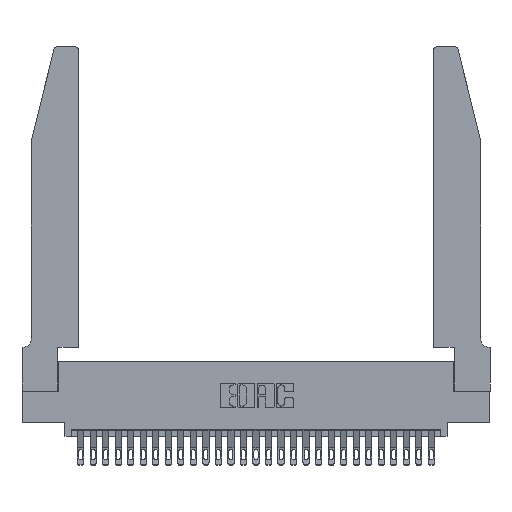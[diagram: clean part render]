
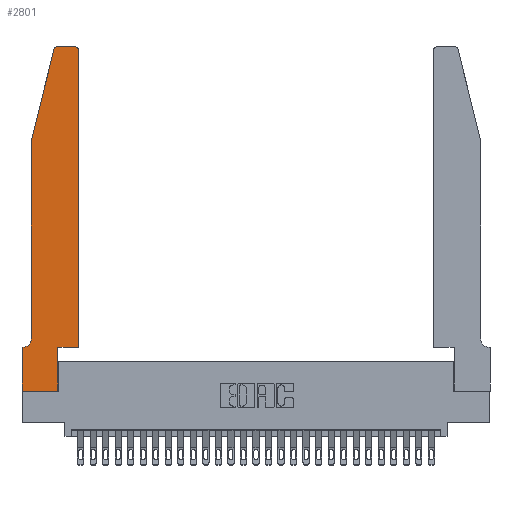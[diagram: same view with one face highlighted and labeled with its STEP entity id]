
A CAD part, top view. The second image highlights one B-rep face of the part: STEP entity #2801.
In plain terms, the highlighted planar face has unit normal (0, 0, 1).
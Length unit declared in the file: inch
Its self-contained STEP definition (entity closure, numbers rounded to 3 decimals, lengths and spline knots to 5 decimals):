
#7 = ORIENTED_EDGE ( 'NONE', *, *, #25601, .T. ) ;
#226 = LINE ( 'NONE', #25525, #24076 ) ;
#768 = ORIENTED_EDGE ( 'NONE', *, *, #28300, .T. ) ;
#838 = LINE ( 'NONE', #29367, #18623 ) ;
#1245 = VERTEX_POINT ( 'NONE', #4473 ) ;
#1294 = CARTESIAN_POINT ( 'NONE',  ( 0., 0.35, 0.37 ) ) ;
#1443 = ORIENTED_EDGE ( 'NONE', *, *, #9442, .T. ) ;
#1467 = CIRCLE ( 'NONE', #15976, 0.03 ) ;
#1729 = LINE ( 'NONE', #11556, #25465 ) ;
#2020 = VERTEX_POINT ( 'NONE', #29300 ) ;
#2185 = EDGE_CURVE ( 'NONE', #14239, #5493, #1467, .T. ) ;
#2212 = DIRECTION ( 'NONE',  ( 1., 0., 0. ) ) ;
#2456 = LINE ( 'NONE', #15847, #26189 ) ;
#2593 = CARTESIAN_POINT ( 'NONE',  ( 0.0055, 0.35, 0.37 ) ) ;
#2801 = ADVANCED_FACE ( 'NONE', ( #16003 ), #4503, .T. ) ;
#2976 = DIRECTION ( 'NONE',  ( -1., 0., 0. ) ) ;
#2997 = CIRCLE ( 'NONE', #26311, 0.07 ) ;
#3949 = DIRECTION ( 'NONE',  ( 0., 1., 0. ) ) ;
#4019 = VERTEX_POINT ( 'NONE', #22606 ) ;
#4306 = ORIENTED_EDGE ( 'NONE', *, *, #5195, .T. ) ;
#4473 = CARTESIAN_POINT ( 'NONE',  ( 0.25487, 2.72718, 0.37 ) ) ;
#4503 = PLANE ( 'NONE',  #16356 ) ;
#4571 = DIRECTION ( 'NONE',  ( 0., 0., -1. ) ) ;
#4838 = DIRECTION ( 'NONE',  ( 0., 0., 1. ) ) ;
#4983 = VECTOR ( 'NONE', #3949, 39.37008 ) ;
#5195 = EDGE_CURVE ( 'NONE', #20004, #14239, #17263, .T. ) ;
#5493 = VERTEX_POINT ( 'NONE', #7193 ) ;
#5931 = CARTESIAN_POINT ( 'NONE',  ( 0.2865, 0., 0.37 ) ) ;
#6699 = DIRECTION ( 'NONE',  ( -1., 0., 0. ) ) ;
#6906 = VERTEX_POINT ( 'NONE', #2593 ) ;
#7050 = DIRECTION ( 'NONE',  ( 1., 0., 0. ) ) ;
#7193 = CARTESIAN_POINT ( 'NONE',  ( 0.4205, 2.75, 0.37 ) ) ;
#7269 = EDGE_CURVE ( 'NONE', #10638, #6906, #2997, .T. ) ;
#8302 = ORIENTED_EDGE ( 'NONE', *, *, #29014, .T. ) ;
#8528 = ORIENTED_EDGE ( 'NONE', *, *, #25649, .T. ) ;
#8791 = DIRECTION ( 'NONE',  ( 0., 0., 1. ) ) ;
#9200 = VERTEX_POINT ( 'NONE', #1294 ) ;
#9442 = EDGE_CURVE ( 'NONE', #28990, #10638, #13063, .T. ) ;
#9600 = AXIS2_PLACEMENT_3D ( 'NONE', #22515, #8791, #24797 ) ;
#10458 = CARTESIAN_POINT ( 'NONE',  ( 0.0755, 2., 0.37 ) ) ;
#10638 = VERTEX_POINT ( 'NONE', #23480 ) ;
#10659 = CARTESIAN_POINT ( 'NONE',  ( 0.4505, 0.35, 0.37 ) ) ;
#11213 = ORIENTED_EDGE ( 'NONE', *, *, #7269, .T. ) ;
#11380 = VECTOR ( 'NONE', #11566, 39.37008 ) ;
#11386 = CARTESIAN_POINT ( 'NONE',  ( 0., 0., 0.37 ) ) ;
#11556 = CARTESIAN_POINT ( 'NONE',  ( 0.4505, 0.35, 0.37 ) ) ;
#11566 = DIRECTION ( 'NONE',  ( 0., -1., 0. ) ) ;
#11785 = ORIENTED_EDGE ( 'NONE', *, *, #18277, .T. ) ;
#12204 = CARTESIAN_POINT ( 'NONE',  ( 0.2605, 2.75, 0.37 ) ) ;
#13063 = LINE ( 'NONE', #25142, #24503 ) ;
#13519 = ORIENTED_EDGE ( 'NONE', *, *, #2185, .T. ) ;
#14164 = DIRECTION ( 'NONE',  ( 1., 0., 0. ) ) ;
#14239 = VERTEX_POINT ( 'NONE', #18963 ) ;
#14609 = LINE ( 'NONE', #10458, #25311 ) ;
#15847 = CARTESIAN_POINT ( 'NONE',  ( 0.0755, 0.35, 0.37 ) ) ;
#15940 = ORIENTED_EDGE ( 'NONE', *, *, #27894, .T. ) ;
#15976 = AXIS2_PLACEMENT_3D ( 'NONE', #18655, #4838, #20942 ) ;
#16003 = FACE_OUTER_BOUND ( 'NONE', #17882, .T. ) ;
#16101 = DIRECTION ( 'NONE',  ( 0., 0., 1. ) ) ;
#16356 = AXIS2_PLACEMENT_3D ( 'NONE', #27390, #16101, #2212 ) ;
#17263 = LINE ( 'NONE', #19996, #4983 ) ;
#17585 = ORIENTED_EDGE ( 'NONE', *, *, #21412, .T. ) ;
#17649 = LINE ( 'NONE', #12204, #22959 ) ;
#17882 = EDGE_LOOP ( 'NONE', ( #29454, #8302, #768, #1443, #11213, #11785, #17585, #8528, #15940, #7, #4306, #13519 ) ) ;
#18277 = EDGE_CURVE ( 'NONE', #6906, #9200, #2456, .T. ) ;
#18393 = CARTESIAN_POINT ( 'NONE',  ( 0.0055, 0.42, 0.37 ) ) ;
#18623 = VECTOR ( 'NONE', #22680, 39.37008 ) ;
#18655 = CARTESIAN_POINT ( 'NONE',  ( 0.4205, 2.72, 0.37 ) ) ;
#18963 = CARTESIAN_POINT ( 'NONE',  ( 0.4505, 2.72, 0.37 ) ) ;
#19105 = EDGE_CURVE ( 'NONE', #5493, #2020, #17649, .T. ) ;
#19996 = CARTESIAN_POINT ( 'NONE',  ( 0.4505, 0.35, 0.37 ) ) ;
#20004 = VERTEX_POINT ( 'NONE', #10659 ) ;
#20158 = CARTESIAN_POINT ( 'NONE',  ( 0.0755, 2., 0.37 ) ) ;
#20678 = DIRECTION ( 'NONE',  ( -1., 0., 0. ) ) ;
#20942 = DIRECTION ( 'NONE',  ( 1., 0., 0. ) ) ;
#21412 = EDGE_CURVE ( 'NONE', #9200, #21655, #23543, .T. ) ;
#21655 = VERTEX_POINT ( 'NONE', #28401 ) ;
#22515 = CARTESIAN_POINT ( 'NONE',  ( 0.284, 2.72, 0.37 ) ) ;
#22606 = CARTESIAN_POINT ( 'NONE',  ( 0.2865, 0.35, 0.37 ) ) ;
#22680 = DIRECTION ( 'NONE',  ( 0., 1., 0. ) ) ;
#22959 = VECTOR ( 'NONE', #2976, 39.37008 ) ;
#23480 = CARTESIAN_POINT ( 'NONE',  ( 0.0755, 0.42, 0.37 ) ) ;
#23543 = LINE ( 'NONE', #11386, #11380 ) ;
#24076 = VECTOR ( 'NONE', #14164, 39.37008 ) ;
#24229 = CIRCLE ( 'NONE', #9600, 0.03 ) ;
#24503 = VECTOR ( 'NONE', #27379, 39.37008 ) ;
#24797 = DIRECTION ( 'NONE',  ( 1., 0., 0. ) ) ;
#25142 = CARTESIAN_POINT ( 'NONE',  ( 0.0755, 2., 0.37 ) ) ;
#25311 = VECTOR ( 'NONE', #26394, 39.37008 ) ;
#25465 = VECTOR ( 'NONE', #7050, 39.37008 ) ;
#25525 = CARTESIAN_POINT ( 'NONE',  ( 0., 0., 0.37 ) ) ;
#25601 = EDGE_CURVE ( 'NONE', #4019, #20004, #1729, .T. ) ;
#25649 = EDGE_CURVE ( 'NONE', #21655, #28317, #226, .T. ) ;
#26189 = VECTOR ( 'NONE', #6699, 39.37008 ) ;
#26311 = AXIS2_PLACEMENT_3D ( 'NONE', #18393, #4571, #20678 ) ;
#26394 = DIRECTION ( 'NONE',  ( -0.239, -0.971, 0. ) ) ;
#27379 = DIRECTION ( 'NONE',  ( 0., -1., 0. ) ) ;
#27390 = CARTESIAN_POINT ( 'NONE',  ( 0., 0.35, 0.37 ) ) ;
#27894 = EDGE_CURVE ( 'NONE', #28317, #4019, #838, .T. ) ;
#28300 = EDGE_CURVE ( 'NONE', #1245, #28990, #14609, .T. ) ;
#28317 = VERTEX_POINT ( 'NONE', #5931 ) ;
#28401 = CARTESIAN_POINT ( 'NONE',  ( 0., 0., 0.37 ) ) ;
#28990 = VERTEX_POINT ( 'NONE', #20158 ) ;
#29014 = EDGE_CURVE ( 'NONE', #2020, #1245, #24229, .T. ) ;
#29300 = CARTESIAN_POINT ( 'NONE',  ( 0.284, 2.75, 0.37 ) ) ;
#29367 = CARTESIAN_POINT ( 'NONE',  ( 0.2865, 0.35, 0.37 ) ) ;
#29454 = ORIENTED_EDGE ( 'NONE', *, *, #19105, .T. ) ;
